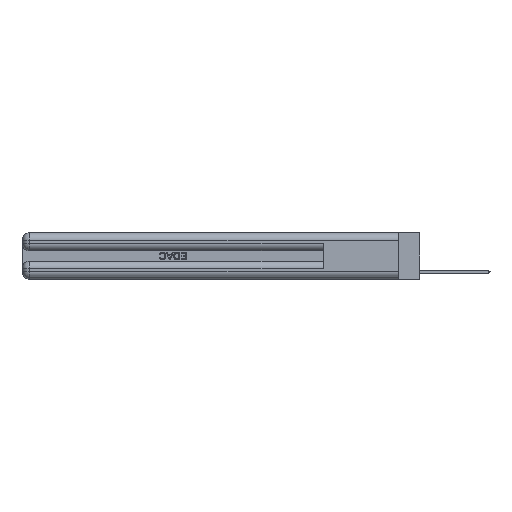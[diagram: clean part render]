
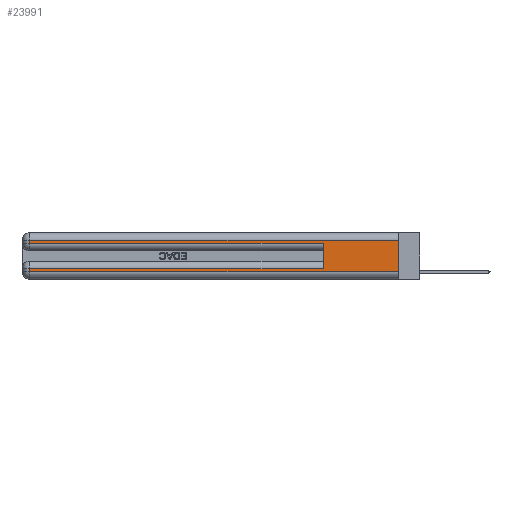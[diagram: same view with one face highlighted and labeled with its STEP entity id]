
A CAD part, left-side view. The second image highlights one B-rep face of the part: STEP entity #23991.
In plain terms, the highlighted planar face has unit normal (-1, 0, 0).
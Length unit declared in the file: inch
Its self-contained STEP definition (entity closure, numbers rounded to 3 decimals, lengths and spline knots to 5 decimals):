
#169 = DIRECTION ( 'NONE',  ( 0., 1., 0. ) ) ;
#884 = LINE ( 'NONE', #24983, #7263 ) ;
#1189 = VECTOR ( 'NONE', #169, 39.37008 ) ;
#1432 = ORIENTED_EDGE ( 'NONE', *, *, #18869, .T. ) ;
#1639 = LINE ( 'NONE', #17979, #33006 ) ;
#2834 = EDGE_CURVE ( 'NONE', #11477, #24773, #19104, .T. ) ;
#4213 = CARTESIAN_POINT ( 'NONE',  ( 0., 2.94, 0.37 ) ) ;
#4389 = VERTEX_POINT ( 'NONE', #8950 ) ;
#5319 = DIRECTION ( 'NONE',  ( 0., 0., -1. ) ) ;
#6514 = EDGE_CURVE ( 'NONE', #24773, #11379, #28282, .T. ) ;
#6906 = ORIENTED_EDGE ( 'NONE', *, *, #6514, .T. ) ;
#7214 = CARTESIAN_POINT ( 'NONE',  ( 0., 2.94, 0.31 ) ) ;
#7263 = VECTOR ( 'NONE', #22503, 39.37008 ) ;
#7427 = LINE ( 'NONE', #21282, #23567 ) ;
#8764 = ORIENTED_EDGE ( 'NONE', *, *, #2834, .T. ) ;
#8950 = CARTESIAN_POINT ( 'NONE',  ( 0., 0., 0.06 ) ) ;
#9431 = ORIENTED_EDGE ( 'NONE', *, *, #32069, .F. ) ;
#9882 = DIRECTION ( 'NONE',  ( 0., 0., -1. ) ) ;
#10076 = CARTESIAN_POINT ( 'NONE',  ( 0., 0., 0.06 ) ) ;
#11221 = EDGE_CURVE ( 'NONE', #20344, #18008, #11474, .T. ) ;
#11379 = VERTEX_POINT ( 'NONE', #20086 ) ;
#11474 = LINE ( 'NONE', #32259, #28187 ) ;
#11477 = VERTEX_POINT ( 'NONE', #31183 ) ;
#11786 = DIRECTION ( 'NONE',  ( 0., 1., 0. ) ) ;
#13321 = CARTESIAN_POINT ( 'NONE',  ( 0., 0., 0.085 ) ) ;
#15313 = AXIS2_PLACEMENT_3D ( 'NONE', #29639, #20998, #26651 ) ;
#15882 = PLANE ( 'NONE',  #15313 ) ;
#15960 = ORIENTED_EDGE ( 'NONE', *, *, #30196, .F. ) ;
#16236 = CARTESIAN_POINT ( 'NONE',  ( 0., 0., 0.31 ) ) ;
#17058 = LINE ( 'NONE', #27823, #30742 ) ;
#17587 = VECTOR ( 'NONE', #28645, 39.37008 ) ;
#17979 = CARTESIAN_POINT ( 'NONE',  ( 0., 0., 0.37 ) ) ;
#18008 = VERTEX_POINT ( 'NONE', #29015 ) ;
#18092 = CARTESIAN_POINT ( 'NONE',  ( 0., 2.94, 0.085 ) ) ;
#18101 = EDGE_LOOP ( 'NONE', ( #15960, #33890, #29475, #34639, #9431, #8764, #6906, #1432 ) ) ;
#18869 = EDGE_CURVE ( 'NONE', #11379, #4389, #33496, .T. ) ;
#19104 = LINE ( 'NONE', #13321, #1189 ) ;
#19501 = EDGE_CURVE ( 'NONE', #20951, #20344, #7427, .T. ) ;
#20086 = CARTESIAN_POINT ( 'NONE',  ( 0., 2.94, 0.06 ) ) ;
#20344 = VERTEX_POINT ( 'NONE', #21691 ) ;
#20951 = VERTEX_POINT ( 'NONE', #7214 ) ;
#20998 = DIRECTION ( 'NONE',  ( 1., 0., 0. ) ) ;
#21282 = CARTESIAN_POINT ( 'NONE',  ( 0., 2.94, 0.37 ) ) ;
#21691 = CARTESIAN_POINT ( 'NONE',  ( 0., 2.94, 0.285 ) ) ;
#22503 = DIRECTION ( 'NONE',  ( 0., 0., 1. ) ) ;
#22965 = VECTOR ( 'NONE', #31026, 39.37008 ) ;
#23567 = VECTOR ( 'NONE', #5319, 39.37008 ) ;
#23991 = ADVANCED_FACE ( 'NONE', ( #31905 ), #15882, .F. ) ;
#24353 = DIRECTION ( 'NONE',  ( 0., -1., 0. ) ) ;
#24773 = VERTEX_POINT ( 'NONE', #18092 ) ;
#24983 = CARTESIAN_POINT ( 'NONE',  ( 0., 0.6, 0.145 ) ) ;
#25324 = VERTEX_POINT ( 'NONE', #16236 ) ;
#26651 = DIRECTION ( 'NONE',  ( 0., 0., -1. ) ) ;
#27823 = CARTESIAN_POINT ( 'NONE',  ( 0., 0., 0.31 ) ) ;
#28187 = VECTOR ( 'NONE', #24353, 39.37008 ) ;
#28225 = EDGE_CURVE ( 'NONE', #25324, #20951, #17058, .T. ) ;
#28282 = LINE ( 'NONE', #4213, #17587 ) ;
#28645 = DIRECTION ( 'NONE',  ( 0., 0., -1. ) ) ;
#29015 = CARTESIAN_POINT ( 'NONE',  ( 0., 0.6, 0.285 ) ) ;
#29475 = ORIENTED_EDGE ( 'NONE', *, *, #19501, .T. ) ;
#29639 = CARTESIAN_POINT ( 'NONE',  ( 0., 0., 0.37 ) ) ;
#30196 = EDGE_CURVE ( 'NONE', #25324, #4389, #1639, .T. ) ;
#30742 = VECTOR ( 'NONE', #11786, 39.37008 ) ;
#31026 = DIRECTION ( 'NONE',  ( 0., -1., 0. ) ) ;
#31183 = CARTESIAN_POINT ( 'NONE',  ( 0., 0.6, 0.085 ) ) ;
#31905 = FACE_OUTER_BOUND ( 'NONE', #18101, .T. ) ;
#32069 = EDGE_CURVE ( 'NONE', #11477, #18008, #884, .T. ) ;
#32259 = CARTESIAN_POINT ( 'NONE',  ( 0., 0., 0.285 ) ) ;
#33006 = VECTOR ( 'NONE', #9882, 39.37008 ) ;
#33496 = LINE ( 'NONE', #10076, #22965 ) ;
#33890 = ORIENTED_EDGE ( 'NONE', *, *, #28225, .T. ) ;
#34639 = ORIENTED_EDGE ( 'NONE', *, *, #11221, .T. ) ;
